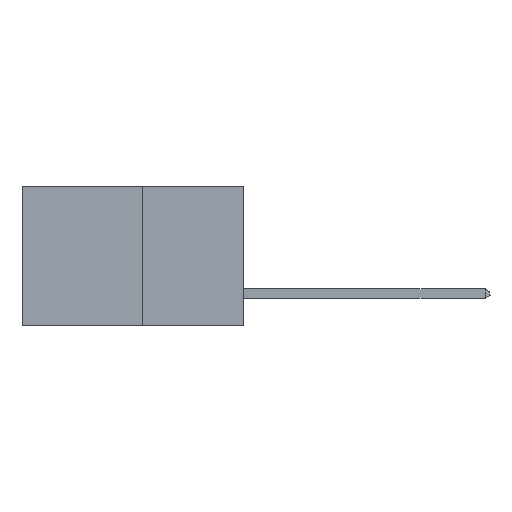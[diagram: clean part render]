
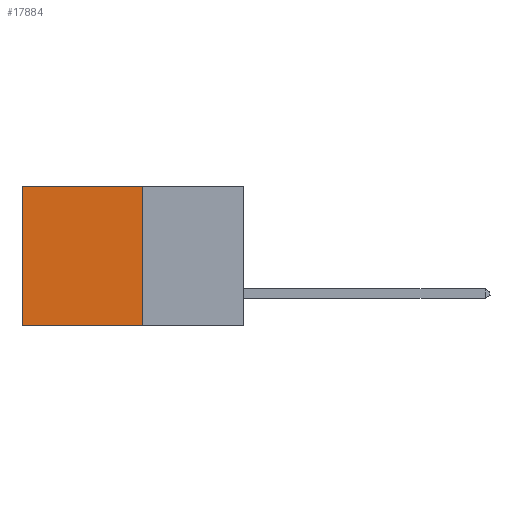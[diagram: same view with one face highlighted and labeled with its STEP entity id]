
A CAD part, left-side view. The second image highlights one B-rep face of the part: STEP entity #17884.
In plain terms, the highlighted planar face has unit normal (-1, 0, 0).
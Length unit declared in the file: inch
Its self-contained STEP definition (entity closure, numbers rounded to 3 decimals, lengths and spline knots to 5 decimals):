
#1255 = EDGE_LOOP ( 'NONE', ( #12774, #8203, #3153, #12641 ) ) ;
#1908 = EDGE_CURVE ( 'NONE', #19483, #4738, #4076, .T. ) ;
#3153 = ORIENTED_EDGE ( 'NONE', *, *, #12493, .F. ) ;
#4076 = LINE ( 'NONE', #10789, #15811 ) ;
#4299 = AXIS2_PLACEMENT_3D ( 'NONE', #18664, #15632, #6079 ) ;
#4459 = PLANE ( 'NONE',  #4299 ) ;
#4738 = VERTEX_POINT ( 'NONE', #18039 ) ;
#4836 = VERTEX_POINT ( 'NONE', #16910 ) ;
#5045 = DIRECTION ( 'NONE',  ( 0., 0., -1. ) ) ;
#5153 = DIRECTION ( 'NONE',  ( 0., 1., 0. ) ) ;
#5232 = CARTESIAN_POINT ( 'NONE',  ( 0.277, 0.27, -0.37 ) ) ;
#5926 = VECTOR ( 'NONE', #5045, 39.37008 ) ;
#6079 = DIRECTION ( 'NONE',  ( 0., 0., -1. ) ) ;
#6656 = FACE_OUTER_BOUND ( 'NONE', #1255, .T. ) ;
#6664 = VECTOR ( 'NONE', #5153, 39.37008 ) ;
#7340 = VERTEX_POINT ( 'NONE', #16690 ) ;
#8203 = ORIENTED_EDGE ( 'NONE', *, *, #8606, .F. ) ;
#8236 = DIRECTION ( 'NONE',  ( 0., 0., -1. ) ) ;
#8606 = EDGE_CURVE ( 'NONE', #4836, #4738, #19759, .T. ) ;
#9949 = CARTESIAN_POINT ( 'NONE',  ( 0.277, 0.59, 0. ) ) ;
#10324 = LINE ( 'NONE', #16985, #18237 ) ;
#10789 = CARTESIAN_POINT ( 'NONE',  ( 0.277, 0.59, -0.37 ) ) ;
#12493 = EDGE_CURVE ( 'NONE', #7340, #4836, #13925, .T. ) ;
#12641 = ORIENTED_EDGE ( 'NONE', *, *, #14373, .T. ) ;
#12774 = ORIENTED_EDGE ( 'NONE', *, *, #1908, .T. ) ;
#13925 = LINE ( 'NONE', #14600, #5926 ) ;
#14373 = EDGE_CURVE ( 'NONE', #7340, #19483, #10324, .T. ) ;
#14600 = CARTESIAN_POINT ( 'NONE',  ( 0.277, 0.27, -0.37 ) ) ;
#15632 = DIRECTION ( 'NONE',  ( 1., 0., 0. ) ) ;
#15811 = VECTOR ( 'NONE', #8236, 39.37008 ) ;
#16690 = CARTESIAN_POINT ( 'NONE',  ( 0.277, 0.27, 0. ) ) ;
#16910 = CARTESIAN_POINT ( 'NONE',  ( 0.277, 0.27, -0.37 ) ) ;
#16985 = CARTESIAN_POINT ( 'NONE',  ( 0.277, 0.27, 0. ) ) ;
#17884 = ADVANCED_FACE ( 'NONE', ( #6656 ), #4459, .F. ) ;
#18039 = CARTESIAN_POINT ( 'NONE',  ( 0.277, 0.59, -0.37 ) ) ;
#18237 = VECTOR ( 'NONE', #18530, 39.37008 ) ;
#18530 = DIRECTION ( 'NONE',  ( 0., 1., 0. ) ) ;
#18664 = CARTESIAN_POINT ( 'NONE',  ( 0.277, 0.27, -0.37 ) ) ;
#19483 = VERTEX_POINT ( 'NONE', #9949 ) ;
#19759 = LINE ( 'NONE', #5232, #6664 ) ;
